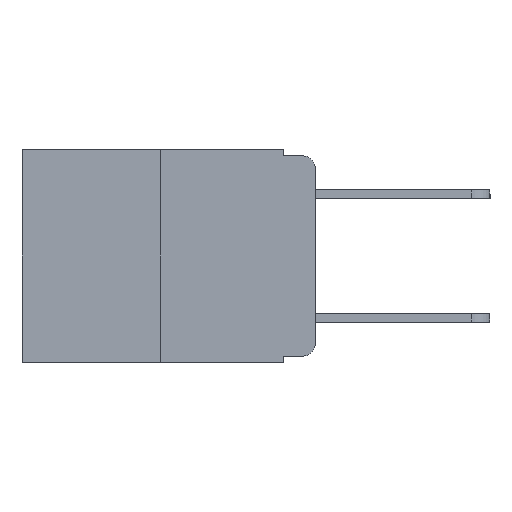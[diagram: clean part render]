
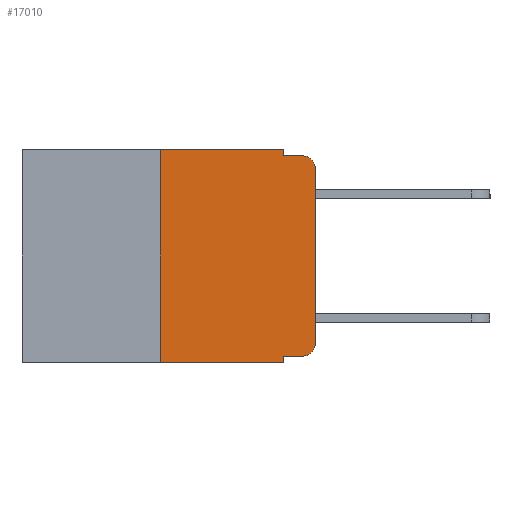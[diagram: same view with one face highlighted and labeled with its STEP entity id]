
A CAD part, left-side view. The second image highlights one B-rep face of the part: STEP entity #17010.
In plain terms, the highlighted planar face has unit normal (-1, 0, 0).
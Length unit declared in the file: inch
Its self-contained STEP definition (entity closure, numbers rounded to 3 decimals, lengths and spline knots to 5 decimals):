
#68 = VERTEX_POINT ( 'NONE', #17271 ) ;
#544 = AXIS2_PLACEMENT_3D ( 'NONE', #20307, #8115, #22342 ) ;
#662 = DIRECTION ( 'NONE',  ( 0., 0., -1. ) ) ;
#1370 = CARTESIAN_POINT ( 'NONE',  ( 0., 0., 0. ) ) ;
#1559 = DIRECTION ( 'NONE',  ( 0., 0., -1. ) ) ;
#2064 = CARTESIAN_POINT ( 'NONE',  ( 0., 0.051, 0. ) ) ;
#2079 = ORIENTED_EDGE ( 'NONE', *, *, #19433, .T. ) ;
#3109 = LINE ( 'NONE', #1370, #7966 ) ;
#3176 = CARTESIAN_POINT ( 'NONE',  ( 0., 0.051, -0.343 ) ) ;
#3497 = DIRECTION ( 'NONE',  ( 0., 0., 1. ) ) ;
#3516 = CARTESIAN_POINT ( 'NONE',  ( 0., 0.473, 0. ) ) ;
#4952 = ORIENTED_EDGE ( 'NONE', *, *, #26597, .F. ) ;
#5102 = EDGE_CURVE ( 'NONE', #68, #16282, #15503, .T. ) ;
#5788 = DIRECTION ( 'NONE',  ( 0., -1., 0. ) ) ;
#6160 = ORIENTED_EDGE ( 'NONE', *, *, #5102, .F. ) ;
#6809 = LINE ( 'NONE', #25271, #21141 ) ;
#7033 = VERTEX_POINT ( 'NONE', #20950 ) ;
#7756 = CARTESIAN_POINT ( 'NONE',  ( 0., 0.051, 0. ) ) ;
#7794 = VECTOR ( 'NONE', #14256, 39.37008 ) ;
#7886 = VERTEX_POINT ( 'NONE', #7756 ) ;
#7966 = VECTOR ( 'NONE', #3497, 39.37008 ) ;
#8021 = EDGE_CURVE ( 'NONE', #10473, #12701, #18596, .T. ) ;
#8065 = AXIS2_PLACEMENT_3D ( 'NONE', #25232, #13101, #662 ) ;
#8115 = DIRECTION ( 'NONE',  ( -1., 0., 0. ) ) ;
#8542 = VECTOR ( 'NONE', #17895, 39.37008 ) ;
#8800 = CARTESIAN_POINT ( 'NONE',  ( 0., 0.051, -0.01 ) ) ;
#9003 = ORIENTED_EDGE ( 'NONE', *, *, #26106, .T. ) ;
#9292 = VECTOR ( 'NONE', #1559, 39.37008 ) ;
#9411 = EDGE_CURVE ( 'NONE', #7886, #10473, #25499, .T. ) ;
#9529 = CARTESIAN_POINT ( 'NONE',  ( 0., 0.25, 0. ) ) ;
#9723 = DIRECTION ( 'NONE',  ( 1., 0., 0. ) ) ;
#10417 = VECTOR ( 'NONE', #22005, 39.37008 ) ;
#10473 = VERTEX_POINT ( 'NONE', #8800 ) ;
#10662 = AXIS2_PLACEMENT_3D ( 'NONE', #3516, #9723, #23955 ) ;
#11053 = DIRECTION ( 'NONE',  ( 0., -1., 0. ) ) ;
#11441 = LINE ( 'NONE', #17918, #10417 ) ;
#11628 = EDGE_CURVE ( 'NONE', #68, #24476, #11441, .T. ) ;
#11851 = ORIENTED_EDGE ( 'NONE', *, *, #11628, .T. ) ;
#12497 = CIRCLE ( 'NONE', #8065, 0.02 ) ;
#12701 = VERTEX_POINT ( 'NONE', #25230 ) ;
#12843 = CARTESIAN_POINT ( 'NONE',  ( 0., 0.02, -0.333 ) ) ;
#13101 = DIRECTION ( 'NONE',  ( -1., 0., 0. ) ) ;
#13378 = EDGE_LOOP ( 'NONE', ( #2079, #26251, #23297, #18600, #20352, #4952, #21739, #6160, #11851, #9003 ) ) ;
#13466 = EDGE_CURVE ( 'NONE', #23750, #7886, #6809, .T. ) ;
#13496 = VECTOR ( 'NONE', #5788, 39.37008 ) ;
#13965 = LINE ( 'NONE', #21895, #8542 ) ;
#14256 = DIRECTION ( 'NONE',  ( 0., -1., 0. ) ) ;
#14388 = DIRECTION ( 'NONE',  ( 0., 0., -1. ) ) ;
#14552 = VERTEX_POINT ( 'NONE', #23293 ) ;
#15315 = EDGE_CURVE ( 'NONE', #20730, #16282, #24283, .T. ) ;
#15503 = LINE ( 'NONE', #2064, #25658 ) ;
#16282 = VERTEX_POINT ( 'NONE', #3176 ) ;
#17010 = ADVANCED_FACE ( 'NONE', ( #20489 ), #21907, .F. ) ;
#17271 = CARTESIAN_POINT ( 'NONE',  ( 0., 0.051, -0.333 ) ) ;
#17895 = DIRECTION ( 'NONE',  ( 0., 0., 1. ) ) ;
#17918 = CARTESIAN_POINT ( 'NONE',  ( 0., 0.051, -0.333 ) ) ;
#18596 = LINE ( 'NONE', #20378, #7794 ) ;
#18600 = ORIENTED_EDGE ( 'NONE', *, *, #9411, .F. ) ;
#19433 = EDGE_CURVE ( 'NONE', #14552, #7033, #3109, .T. ) ;
#20041 = CARTESIAN_POINT ( 'NONE',  ( 0., 0.473, -0.343 ) ) ;
#20307 = CARTESIAN_POINT ( 'NONE',  ( 0., 0.02, -0.313 ) ) ;
#20352 = ORIENTED_EDGE ( 'NONE', *, *, #13466, .F. ) ;
#20378 = CARTESIAN_POINT ( 'NONE',  ( 0., 0.051, -0.01 ) ) ;
#20489 = FACE_OUTER_BOUND ( 'NONE', #13378, .T. ) ;
#20730 = VERTEX_POINT ( 'NONE', #25747 ) ;
#20950 = CARTESIAN_POINT ( 'NONE',  ( 0., 0., -0.03 ) ) ;
#21141 = VECTOR ( 'NONE', #11053, 39.37008 ) ;
#21739 = ORIENTED_EDGE ( 'NONE', *, *, #15315, .T. ) ;
#21895 = CARTESIAN_POINT ( 'NONE',  ( 0., 0.25, 0. ) ) ;
#21907 = PLANE ( 'NONE',  #10662 ) ;
#21997 = CARTESIAN_POINT ( 'NONE',  ( 0., 0.051, 0. ) ) ;
#22005 = DIRECTION ( 'NONE',  ( 0., -1., 0. ) ) ;
#22342 = DIRECTION ( 'NONE',  ( 0., 0., -1. ) ) ;
#23293 = CARTESIAN_POINT ( 'NONE',  ( 0., 0., -0.313 ) ) ;
#23297 = ORIENTED_EDGE ( 'NONE', *, *, #8021, .F. ) ;
#23565 = EDGE_CURVE ( 'NONE', #7033, #12701, #12497, .T. ) ;
#23750 = VERTEX_POINT ( 'NONE', #9529 ) ;
#23955 = DIRECTION ( 'NONE',  ( 0., 0., -1. ) ) ;
#24283 = LINE ( 'NONE', #20041, #13496 ) ;
#24476 = VERTEX_POINT ( 'NONE', #12843 ) ;
#25230 = CARTESIAN_POINT ( 'NONE',  ( 0., 0.02, -0.01 ) ) ;
#25232 = CARTESIAN_POINT ( 'NONE',  ( 0., 0.02, -0.03 ) ) ;
#25271 = CARTESIAN_POINT ( 'NONE',  ( 0., 0.473, 0. ) ) ;
#25499 = LINE ( 'NONE', #21997, #9292 ) ;
#25658 = VECTOR ( 'NONE', #14388, 39.37008 ) ;
#25747 = CARTESIAN_POINT ( 'NONE',  ( 0., 0.25, -0.343 ) ) ;
#26080 = CIRCLE ( 'NONE', #544, 0.02 ) ;
#26106 = EDGE_CURVE ( 'NONE', #24476, #14552, #26080, .T. ) ;
#26251 = ORIENTED_EDGE ( 'NONE', *, *, #23565, .T. ) ;
#26597 = EDGE_CURVE ( 'NONE', #20730, #23750, #13965, .T. ) ;
